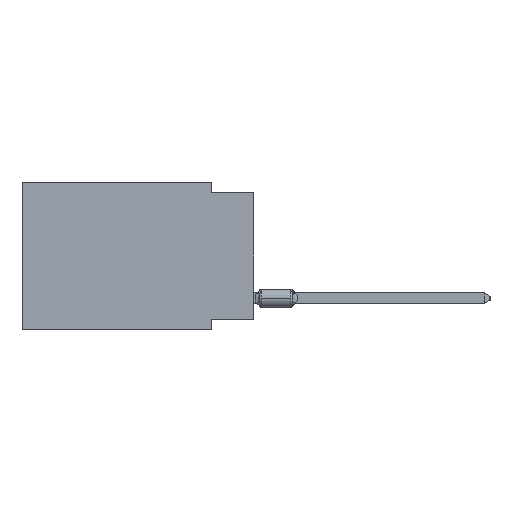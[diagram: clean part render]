
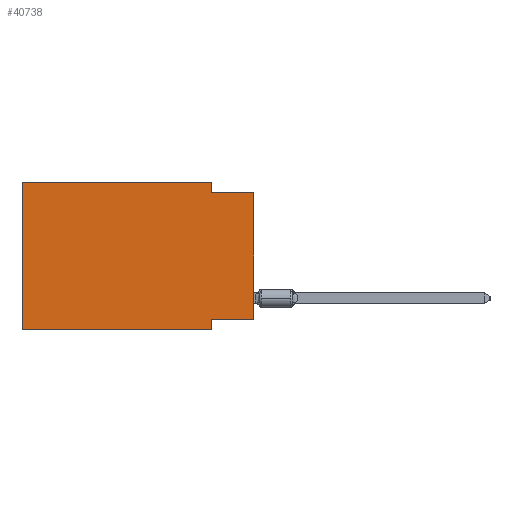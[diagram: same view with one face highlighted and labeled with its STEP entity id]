
A CAD part, left-side view. The second image highlights one B-rep face of the part: STEP entity #40738.
In plain terms, the highlighted planar face has unit normal (-1, 0, 0).
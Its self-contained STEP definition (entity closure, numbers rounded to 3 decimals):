
#427 = CARTESIAN_POINT ( 'NONE',  ( 0., 0., -8.255 ) ) ;
#1237 = CARTESIAN_POINT ( 'NONE',  ( 0., 13.97, 0. ) ) ;
#1407 = VERTEX_POINT ( 'NONE', #52650 ) ;
#1601 = CARTESIAN_POINT ( 'NONE',  ( 0., 13.97, 0. ) ) ;
#1999 = EDGE_CURVE ( 'NONE', #45360, #49037, #33032, .T. ) ;
#2436 = VECTOR ( 'NONE', #33585, 1000. ) ;
#4151 = ORIENTED_EDGE ( 'NONE', *, *, #6366, .T. ) ;
#4698 = CARTESIAN_POINT ( 'NONE',  ( 0., 13.97, 0. ) ) ;
#5012 = ORIENTED_EDGE ( 'NONE', *, *, #8516, .F. ) ;
#5675 = CARTESIAN_POINT ( 'NONE',  ( 0., 2.54, -0.635 ) ) ;
#5687 = VERTEX_POINT ( 'NONE', #24963 ) ;
#5789 = VECTOR ( 'NONE', #16674, 1000. ) ;
#6366 = EDGE_CURVE ( 'NONE', #17536, #19761, #24777, .T. ) ;
#7280 = AXIS2_PLACEMENT_3D ( 'NONE', #24538, #48784, #43731 ) ;
#7512 = DIRECTION ( 'NONE',  ( 0., -1., 0. ) ) ;
#7777 = LINE ( 'NONE', #27741, #29189 ) ;
#7944 = LINE ( 'NONE', #35900, #29982 ) ;
#8516 = EDGE_CURVE ( 'NONE', #5687, #49149, #36481, .T. ) ;
#9328 = DIRECTION ( 'NONE',  ( 0., 0., 1. ) ) ;
#10384 = ORIENTED_EDGE ( 'NONE', *, *, #33710, .F. ) ;
#11461 = DIRECTION ( 'NONE',  ( 0., 0., -1. ) ) ;
#11987 = CARTESIAN_POINT ( 'NONE',  ( 0., 2.54, -8.89 ) ) ;
#16298 = FACE_OUTER_BOUND ( 'NONE', #46067, .T. ) ;
#16674 = DIRECTION ( 'NONE',  ( 0., 1., 0. ) ) ;
#17490 = DIRECTION ( 'NONE',  ( 0., -1., 0. ) ) ;
#17536 = VERTEX_POINT ( 'NONE', #19720 ) ;
#18281 = LINE ( 'NONE', #1237, #34613 ) ;
#18449 = ORIENTED_EDGE ( 'NONE', *, *, #24505, .F. ) ;
#19720 = CARTESIAN_POINT ( 'NONE',  ( 0., 0., -8.255 ) ) ;
#19761 = VERTEX_POINT ( 'NONE', #36866 ) ;
#21345 = CARTESIAN_POINT ( 'NONE',  ( 0., 2.54, 0. ) ) ;
#21455 = CARTESIAN_POINT ( 'NONE',  ( 0., 2.54, -8.89 ) ) ;
#21602 = EDGE_CURVE ( 'NONE', #1407, #49676, #25864, .T. ) ;
#24505 = EDGE_CURVE ( 'NONE', #49676, #19761, #7944, .T. ) ;
#24520 = ORIENTED_EDGE ( 'NONE', *, *, #43563, .T. ) ;
#24538 = CARTESIAN_POINT ( 'NONE',  ( 0., 13.97, 0. ) ) ;
#24777 = LINE ( 'NONE', #36247, #37080 ) ;
#24963 = CARTESIAN_POINT ( 'NONE',  ( 0., 2.54, -8.255 ) ) ;
#25864 = LINE ( 'NONE', #21345, #2436 ) ;
#27741 = CARTESIAN_POINT ( 'NONE',  ( 0., 13.97, -8.89 ) ) ;
#28967 = EDGE_CURVE ( 'NONE', #17536, #5687, #32890, .T. ) ;
#29189 = VECTOR ( 'NONE', #7512, 1000. ) ;
#29766 = CARTESIAN_POINT ( 'NONE',  ( 0., 13.97, -8.89 ) ) ;
#29982 = VECTOR ( 'NONE', #36689, 1000. ) ;
#32890 = LINE ( 'NONE', #427, #5789 ) ;
#33032 = LINE ( 'NONE', #1601, #42033 ) ;
#33585 = DIRECTION ( 'NONE',  ( 0., 0., -1. ) ) ;
#33710 = EDGE_CURVE ( 'NONE', #49037, #1407, #18281, .T. ) ;
#34613 = VECTOR ( 'NONE', #17490, 1000. ) ;
#35900 = CARTESIAN_POINT ( 'NONE',  ( 0., 0., -0.635 ) ) ;
#36247 = CARTESIAN_POINT ( 'NONE',  ( 0., 0., 0. ) ) ;
#36481 = LINE ( 'NONE', #11987, #42323 ) ;
#36689 = DIRECTION ( 'NONE',  ( 0., -1., 0. ) ) ;
#36774 = PLANE ( 'NONE',  #7280 ) ;
#36866 = CARTESIAN_POINT ( 'NONE',  ( 0., 0., -0.635 ) ) ;
#37080 = VECTOR ( 'NONE', #41277, 1000. ) ;
#40738 = ADVANCED_FACE ( 'NONE', ( #16298 ), #36774, .F. ) ;
#41277 = DIRECTION ( 'NONE',  ( 0., 0., 1. ) ) ;
#41921 = ORIENTED_EDGE ( 'NONE', *, *, #1999, .F. ) ;
#42033 = VECTOR ( 'NONE', #9328, 1000. ) ;
#42323 = VECTOR ( 'NONE', #11461, 1000. ) ;
#43563 = EDGE_CURVE ( 'NONE', #45360, #49149, #7777, .T. ) ;
#43731 = DIRECTION ( 'NONE',  ( 0., 0., -1. ) ) ;
#45360 = VERTEX_POINT ( 'NONE', #29766 ) ;
#45593 = ORIENTED_EDGE ( 'NONE', *, *, #28967, .F. ) ;
#46067 = EDGE_LOOP ( 'NONE', ( #4151, #18449, #46797, #10384, #41921, #24520, #5012, #45593 ) ) ;
#46797 = ORIENTED_EDGE ( 'NONE', *, *, #21602, .F. ) ;
#48784 = DIRECTION ( 'NONE',  ( 1., 0., 0. ) ) ;
#49037 = VERTEX_POINT ( 'NONE', #4698 ) ;
#49149 = VERTEX_POINT ( 'NONE', #21455 ) ;
#49676 = VERTEX_POINT ( 'NONE', #5675 ) ;
#52650 = CARTESIAN_POINT ( 'NONE',  ( 0., 2.54, 0. ) ) ;
